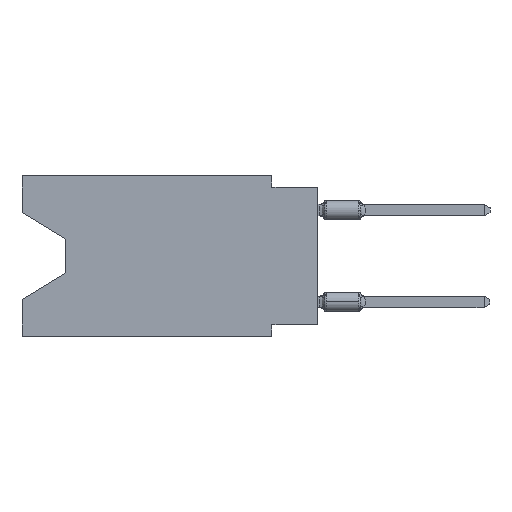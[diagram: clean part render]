
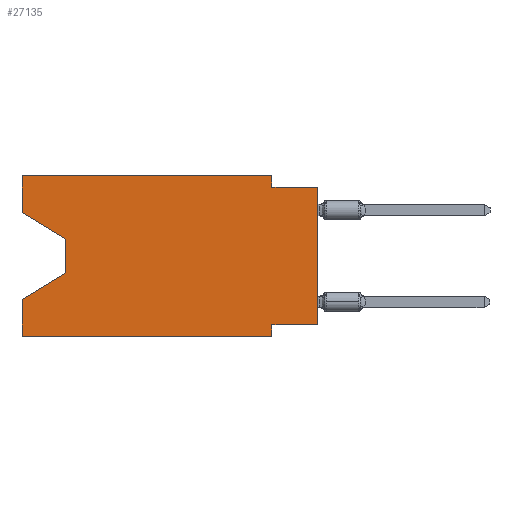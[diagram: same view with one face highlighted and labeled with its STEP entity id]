
A CAD part, left-side view. The second image highlights one B-rep face of the part: STEP entity #27135.
In plain terms, the highlighted planar face has unit normal (-1, 0, 0).
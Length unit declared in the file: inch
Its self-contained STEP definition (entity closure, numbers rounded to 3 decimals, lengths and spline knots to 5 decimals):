
#271 = VECTOR ( 'NONE', #865, 39.37008 ) ;
#711 = CARTESIAN_POINT ( 'NONE',  ( 0., 0.645, 0. ) ) ;
#865 = DIRECTION ( 'NONE',  ( 0., 0., -1. ) ) ;
#1254 = EDGE_LOOP ( 'NONE', ( #20659, #27790, #17561, #13809, #11035, #4245, #25669, #2877, #18337, #24035, #21528, #13301 ) ) ;
#1355 = VERTEX_POINT ( 'NONE', #24272 ) ;
#1747 = FACE_OUTER_BOUND ( 'NONE', #1254, .T. ) ;
#2876 = LINE ( 'NONE', #16287, #20672 ) ;
#2877 = ORIENTED_EDGE ( 'NONE', *, *, #7485, .T. ) ;
#2961 = DIRECTION ( 'NONE',  ( 0., -1., 0. ) ) ;
#3087 = VERTEX_POINT ( 'NONE', #11013 ) ;
#3107 = LINE ( 'NONE', #7424, #12197 ) ;
#3154 = VECTOR ( 'NONE', #28702, 39.37008 ) ;
#3590 = EDGE_CURVE ( 'NONE', #1355, #19239, #3107, .T. ) ;
#3679 = VERTEX_POINT ( 'NONE', #23528 ) ;
#4245 = ORIENTED_EDGE ( 'NONE', *, *, #24981, .F. ) ;
#4266 = VECTOR ( 'NONE', #9218, 39.37008 ) ;
#4378 = CARTESIAN_POINT ( 'NONE',  ( 0., 0., -0.025 ) ) ;
#4714 = VECTOR ( 'NONE', #25770, 39.37008 ) ;
#4957 = VERTEX_POINT ( 'NONE', #6086 ) ;
#6051 = CARTESIAN_POINT ( 'NONE',  ( 0., 0.645, -0.08025 ) ) ;
#6086 = CARTESIAN_POINT ( 'NONE',  ( 0., 0.645, -0.26975 ) ) ;
#6194 = CARTESIAN_POINT ( 'NONE',  ( 0., 0.645, 0. ) ) ;
#6224 = VERTEX_POINT ( 'NONE', #20055 ) ;
#6274 = DIRECTION ( 'NONE',  ( 0., 1., 0. ) ) ;
#6472 = LINE ( 'NONE', #4378, #20993 ) ;
#6582 = LINE ( 'NONE', #15236, #26891 ) ;
#7424 = CARTESIAN_POINT ( 'NONE',  ( 0., 0.645, -0.35 ) ) ;
#7444 = CARTESIAN_POINT ( 'NONE',  ( 0., 0.645, 0. ) ) ;
#7485 = EDGE_CURVE ( 'NONE', #6224, #8593, #22696, .T. ) ;
#7523 = VERTEX_POINT ( 'NONE', #20005 ) ;
#8212 = LINE ( 'NONE', #22087, #25647 ) ;
#8589 = PLANE ( 'NONE',  #11721 ) ;
#8593 = VERTEX_POINT ( 'NONE', #15855 ) ;
#8915 = CARTESIAN_POINT ( 'NONE',  ( 0., 0.55, -0.212 ) ) ;
#9218 = DIRECTION ( 'NONE',  ( 0., 0., -1. ) ) ;
#9334 = VERTEX_POINT ( 'NONE', #25975 ) ;
#11013 = CARTESIAN_POINT ( 'NONE',  ( 0., 0.1, 0. ) ) ;
#11035 = ORIENTED_EDGE ( 'NONE', *, *, #3590, .T. ) ;
#11079 = DIRECTION ( 'NONE',  ( 0., -1., 0. ) ) ;
#11721 = AXIS2_PLACEMENT_3D ( 'NONE', #6194, #24982, #24685 ) ;
#11791 = DIRECTION ( 'NONE',  ( 0., -1., 0. ) ) ;
#12040 = EDGE_CURVE ( 'NONE', #20244, #4957, #13382, .T. ) ;
#12197 = VECTOR ( 'NONE', #2961, 39.37008 ) ;
#12290 = VERTEX_POINT ( 'NONE', #711 ) ;
#12468 = LINE ( 'NONE', #23655, #271 ) ;
#13049 = EDGE_CURVE ( 'NONE', #7523, #8593, #6472, .T. ) ;
#13301 = ORIENTED_EDGE ( 'NONE', *, *, #25306, .F. ) ;
#13382 = LINE ( 'NONE', #8915, #23078 ) ;
#13809 = ORIENTED_EDGE ( 'NONE', *, *, #18651, .F. ) ;
#14603 = LINE ( 'NONE', #7444, #4714 ) ;
#14720 = LINE ( 'NONE', #19332, #28249 ) ;
#15186 = DIRECTION ( 'NONE',  ( 0., 0.855, -0.519 ) ) ;
#15236 = CARTESIAN_POINT ( 'NONE',  ( 0., 0.645, 0. ) ) ;
#15349 = LINE ( 'NONE', #20388, #4266 ) ;
#15855 = CARTESIAN_POINT ( 'NONE',  ( 0., 0., -0.025 ) ) ;
#16287 = CARTESIAN_POINT ( 'NONE',  ( 0., 0.1, -0.35 ) ) ;
#17185 = EDGE_CURVE ( 'NONE', #6224, #20437, #8212, .T. ) ;
#17561 = ORIENTED_EDGE ( 'NONE', *, *, #12040, .T. ) ;
#18314 = CARTESIAN_POINT ( 'NONE',  ( 0., 0.1, -0.35 ) ) ;
#18337 = ORIENTED_EDGE ( 'NONE', *, *, #13049, .F. ) ;
#18528 = CARTESIAN_POINT ( 'NONE',  ( 0., 0.55, -0.212 ) ) ;
#18651 = EDGE_CURVE ( 'NONE', #1355, #4957, #14603, .T. ) ;
#19152 = EDGE_CURVE ( 'NONE', #3087, #7523, #15349, .T. ) ;
#19239 = VERTEX_POINT ( 'NONE', #18314 ) ;
#19332 = CARTESIAN_POINT ( 'NONE',  ( 0., 0.645, 0. ) ) ;
#20005 = CARTESIAN_POINT ( 'NONE',  ( 0., 0.1, -0.025 ) ) ;
#20055 = CARTESIAN_POINT ( 'NONE',  ( 0., 0., -0.325 ) ) ;
#20244 = VERTEX_POINT ( 'NONE', #18528 ) ;
#20388 = CARTESIAN_POINT ( 'NONE',  ( 0., 0.1, 0. ) ) ;
#20437 = VERTEX_POINT ( 'NONE', #24644 ) ;
#20659 = ORIENTED_EDGE ( 'NONE', *, *, #26984, .T. ) ;
#20672 = VECTOR ( 'NONE', #27607, 39.37008 ) ;
#20993 = VECTOR ( 'NONE', #11079, 39.37008 ) ;
#21528 = ORIENTED_EDGE ( 'NONE', *, *, #24388, .F. ) ;
#22087 = CARTESIAN_POINT ( 'NONE',  ( 0., 0., -0.325 ) ) ;
#22696 = LINE ( 'NONE', #27307, #22906 ) ;
#22906 = VECTOR ( 'NONE', #27162, 39.37008 ) ;
#23078 = VECTOR ( 'NONE', #15186, 39.37008 ) ;
#23528 = CARTESIAN_POINT ( 'NONE',  ( 0., 0.55, -0.138 ) ) ;
#23655 = CARTESIAN_POINT ( 'NONE',  ( 0., 0.55, -0.138 ) ) ;
#24035 = ORIENTED_EDGE ( 'NONE', *, *, #19152, .F. ) ;
#24272 = CARTESIAN_POINT ( 'NONE',  ( 0., 0.645, -0.35 ) ) ;
#24388 = EDGE_CURVE ( 'NONE', #12290, #3087, #14720, .T. ) ;
#24644 = CARTESIAN_POINT ( 'NONE',  ( 0., 0.1, -0.325 ) ) ;
#24685 = DIRECTION ( 'NONE',  ( 0., 0., -1. ) ) ;
#24981 = EDGE_CURVE ( 'NONE', #20437, #19239, #2876, .T. ) ;
#24982 = DIRECTION ( 'NONE',  ( 1., 0., 0. ) ) ;
#25306 = EDGE_CURVE ( 'NONE', #9334, #12290, #6582, .T. ) ;
#25647 = VECTOR ( 'NONE', #6274, 39.37008 ) ;
#25669 = ORIENTED_EDGE ( 'NONE', *, *, #17185, .F. ) ;
#25770 = DIRECTION ( 'NONE',  ( 0., 0., 1. ) ) ;
#25975 = CARTESIAN_POINT ( 'NONE',  ( 0., 0.645, -0.08025 ) ) ;
#26045 = EDGE_CURVE ( 'NONE', #3679, #20244, #12468, .T. ) ;
#26704 = DIRECTION ( 'NONE',  ( 0., 0., 1. ) ) ;
#26891 = VECTOR ( 'NONE', #26704, 39.37008 ) ;
#26984 = EDGE_CURVE ( 'NONE', #9334, #3679, #28258, .T. ) ;
#27135 = ADVANCED_FACE ( 'NONE', ( #1747 ), #8589, .F. ) ;
#27162 = DIRECTION ( 'NONE',  ( 0., 0., 1. ) ) ;
#27307 = CARTESIAN_POINT ( 'NONE',  ( 0., 0., 0. ) ) ;
#27607 = DIRECTION ( 'NONE',  ( 0., 0., -1. ) ) ;
#27790 = ORIENTED_EDGE ( 'NONE', *, *, #26045, .T. ) ;
#28249 = VECTOR ( 'NONE', #11791, 39.37008 ) ;
#28258 = LINE ( 'NONE', #6051, #3154 ) ;
#28702 = DIRECTION ( 'NONE',  ( 0., -0.855, -0.519 ) ) ;
